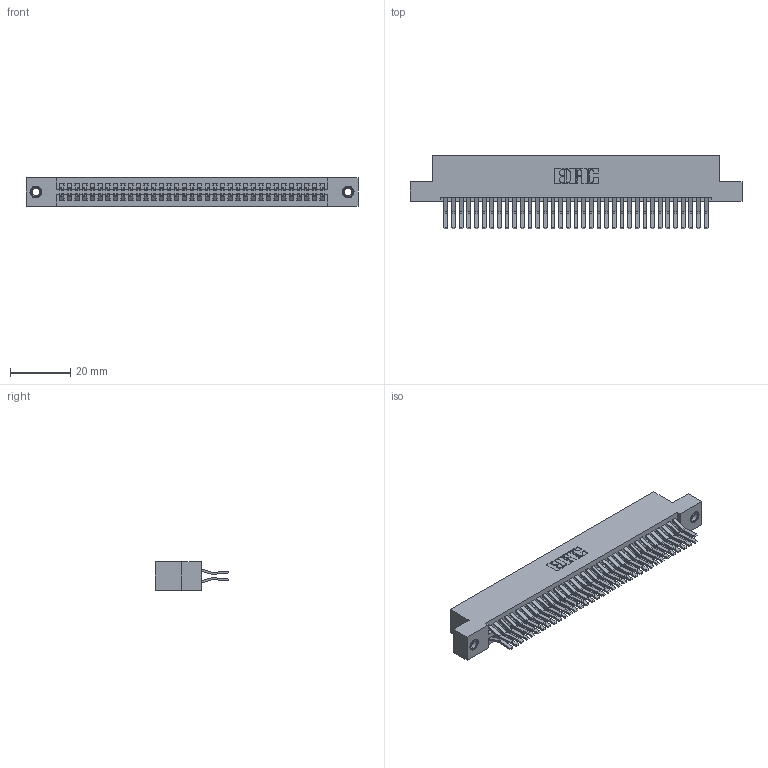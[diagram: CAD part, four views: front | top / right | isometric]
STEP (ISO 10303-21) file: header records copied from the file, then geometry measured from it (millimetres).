
FILE_DESCRIPTION (( 'STEP AP203' ), '1' );
FILE_NAME ('345-070-560-207.STEP', '2018-10-01T11:18:43', ( '' ), ( '' ), 'SwSTEP 2.0', 'SolidWorks 2016', '' );
FILE_SCHEMA (( 'CONFIG_CONTROL_DESIGN' ));
Length unit declared in the file: inch
Products named in the file (4): 345-070-560-207; 345-250-001_345-250-005-103; 345 Part_Flush Mounting Lugs - 0.156 Dia-TI; 345-292-001_560 Tail
Assembly tree (73 placements, depth 2):
  345-070-560-207
    345 Part_Flush Mounting Lugs - 0.156 Dia-TI
    345-292-001_560 Tail  x70
    345-250-001_345-250-005-103  x2
Bounding box: 110.11 x 24.45 x 9.4 mm (x, y, z)
Volume: 11076.4 mm3; surface area: 17445.2 mm2
Topology: 73 solids, 73 shells, 3826 faces, 11327 edges, 7450 vertices
Faces by surface type: plane 2422, cylinder 1388, cone 12, torus 4
Entity records: 29678 total; most frequent: CARTESIAN_POINT 4963, ORIENTED_EDGE 4890, DIRECTION 4415, EDGE_CURVE 2445, VECTOR 2149, LINE 2149, VERTEX_POINT 1624, AXIS2_PLACEMENT_3D 1133
